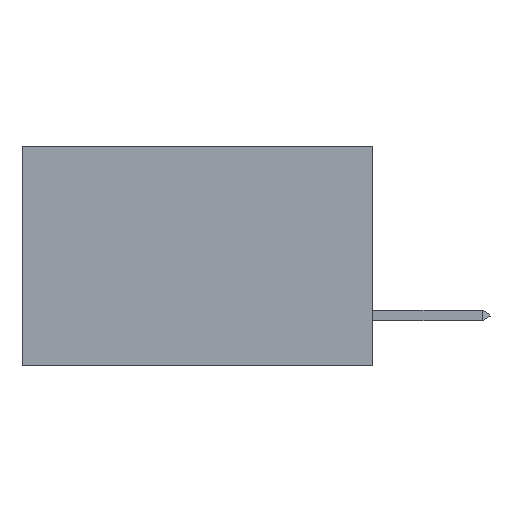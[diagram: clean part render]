
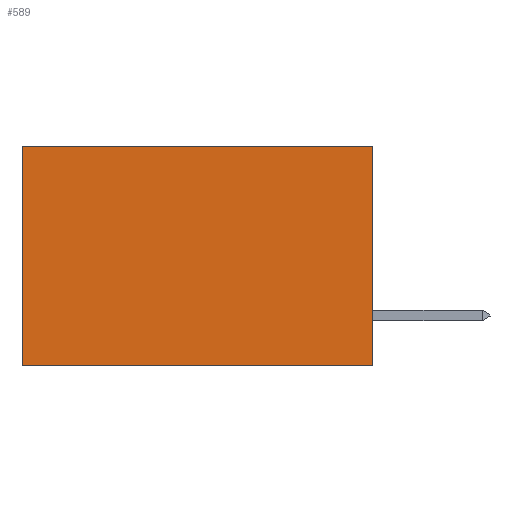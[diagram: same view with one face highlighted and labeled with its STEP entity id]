
A CAD part, left-side view. The second image highlights one B-rep face of the part: STEP entity #589.
In plain terms, the highlighted planar face has unit normal (-1, 0, 0).
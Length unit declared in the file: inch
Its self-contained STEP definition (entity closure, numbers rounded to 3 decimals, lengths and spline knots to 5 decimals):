
#155 = VERTEX_POINT ( 'NONE', #5680 ) ;
#304 = VECTOR ( 'NONE', #2602, 39.37008 ) ;
#589 = ADVANCED_FACE ( 'NONE', ( #10557 ), #5209, .F. ) ;
#647 = LINE ( 'NONE', #12249, #304 ) ;
#659 = VECTOR ( 'NONE', #12848, 39.37008 ) ;
#1124 = EDGE_CURVE ( 'NONE', #155, #8034, #647, .T. ) ;
#1443 = ORIENTED_EDGE ( 'NONE', *, *, #5960, .T. ) ;
#1521 = CARTESIAN_POINT ( 'NONE',  ( 0.277, 0., 0. ) ) ;
#2602 = DIRECTION ( 'NONE',  ( 0., 1., 0. ) ) ;
#2629 = DIRECTION ( 'NONE',  ( 0., 1., 0. ) ) ;
#2787 = DIRECTION ( 'NONE',  ( 0., 0., -1. ) ) ;
#3205 = VERTEX_POINT ( 'NONE', #4596 ) ;
#3560 = LINE ( 'NONE', #11869, #659 ) ;
#3614 = DIRECTION ( 'NONE',  ( 1., 0., 0. ) ) ;
#4411 = CARTESIAN_POINT ( 'NONE',  ( 0.277, 0.59, 0. ) ) ;
#4443 = ORIENTED_EDGE ( 'NONE', *, *, #9127, .T. ) ;
#4596 = CARTESIAN_POINT ( 'NONE',  ( 0.277, 0., 0. ) ) ;
#4837 = VECTOR ( 'NONE', #2629, 39.37008 ) ;
#5018 = LINE ( 'NONE', #6156, #9807 ) ;
#5168 = CARTESIAN_POINT ( 'NONE',  ( 0.277, 0.59, -0.37 ) ) ;
#5209 = PLANE ( 'NONE',  #5240 ) ;
#5240 = AXIS2_PLACEMENT_3D ( 'NONE', #10870, #3614, #2787 ) ;
#5466 = ORIENTED_EDGE ( 'NONE', *, *, #9291, .F. ) ;
#5680 = CARTESIAN_POINT ( 'NONE',  ( 0.277, 0., -0.37 ) ) ;
#5711 = ORIENTED_EDGE ( 'NONE', *, *, #1124, .F. ) ;
#5912 = DIRECTION ( 'NONE',  ( 0., 0., -1. ) ) ;
#5960 = EDGE_CURVE ( 'NONE', #9803, #8034, #5018, .T. ) ;
#6156 = CARTESIAN_POINT ( 'NONE',  ( 0.277, 0.59, -0.37 ) ) ;
#7529 = LINE ( 'NONE', #1521, #4837 ) ;
#8034 = VERTEX_POINT ( 'NONE', #5168 ) ;
#9127 = EDGE_CURVE ( 'NONE', #3205, #9803, #7529, .T. ) ;
#9291 = EDGE_CURVE ( 'NONE', #3205, #155, #3560, .T. ) ;
#9803 = VERTEX_POINT ( 'NONE', #4411 ) ;
#9807 = VECTOR ( 'NONE', #5912, 39.37008 ) ;
#10557 = FACE_OUTER_BOUND ( 'NONE', #12889, .T. ) ;
#10870 = CARTESIAN_POINT ( 'NONE',  ( 0.277, 0., -0.37 ) ) ;
#11869 = CARTESIAN_POINT ( 'NONE',  ( 0.277, 0., -0.37 ) ) ;
#12249 = CARTESIAN_POINT ( 'NONE',  ( 0.277, 0., -0.37 ) ) ;
#12848 = DIRECTION ( 'NONE',  ( 0., 0., -1. ) ) ;
#12889 = EDGE_LOOP ( 'NONE', ( #1443, #5711, #5466, #4443 ) ) ;
